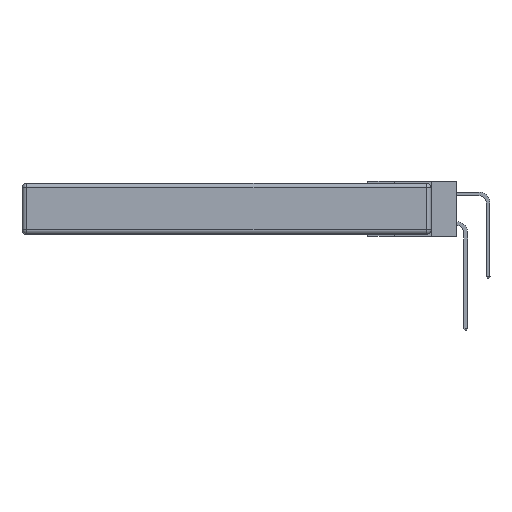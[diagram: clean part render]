
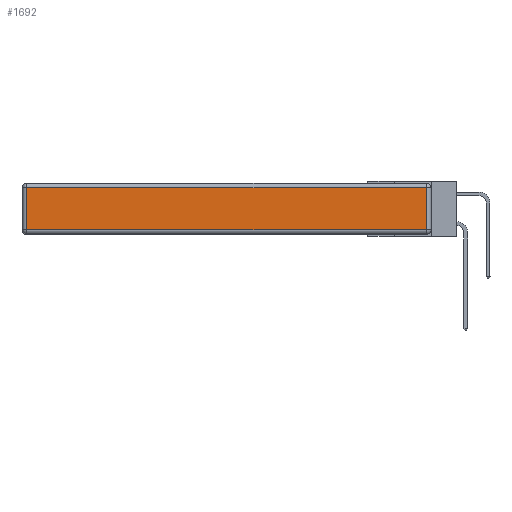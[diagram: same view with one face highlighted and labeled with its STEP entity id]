
A CAD part, left-side view. The second image highlights one B-rep face of the part: STEP entity #1692.
In plain terms, the highlighted planar face has unit normal (-1, 0, 0).
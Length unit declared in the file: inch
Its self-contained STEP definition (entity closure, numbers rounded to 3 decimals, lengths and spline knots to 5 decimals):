
#292 = EDGE_LOOP ( 'NONE', ( #3647, #696, #10602, #1207 ) ) ;
#347 = CARTESIAN_POINT ( 'NONE',  ( 0., 0.03, -0.313 ) ) ;
#696 = ORIENTED_EDGE ( 'NONE', *, *, #6113, .T. ) ;
#996 = PLANE ( 'NONE',  #8773 ) ;
#1207 = ORIENTED_EDGE ( 'NONE', *, *, #12230, .T. ) ;
#1393 = CARTESIAN_POINT ( 'NONE',  ( 0., 0.03, -0.343 ) ) ;
#1673 = DIRECTION ( 'NONE',  ( -1., 0., 0. ) ) ;
#1692 = ADVANCED_FACE ( 'NONE', ( #14883 ), #996, .T. ) ;
#2790 = LINE ( 'NONE', #9106, #5074 ) ;
#3324 = EDGE_CURVE ( 'NONE', #14951, #9114, #3427, .T. ) ;
#3427 = LINE ( 'NONE', #12201, #11537 ) ;
#3623 = VERTEX_POINT ( 'NONE', #14564 ) ;
#3647 = ORIENTED_EDGE ( 'NONE', *, *, #4901, .T. ) ;
#3852 = DIRECTION ( 'NONE',  ( 0., -1., 0. ) ) ;
#4124 = CARTESIAN_POINT ( 'NONE',  ( 0., 0., -0.313 ) ) ;
#4168 = DIRECTION ( 'NONE',  ( 0., 0., 1. ) ) ;
#4195 = CARTESIAN_POINT ( 'NONE',  ( 0., 2.72, -0.03 ) ) ;
#4901 = EDGE_CURVE ( 'NONE', #3623, #14210, #8957, .T. ) ;
#5034 = DIRECTION ( 'NONE',  ( 0., 0., 1. ) ) ;
#5074 = VECTOR ( 'NONE', #14095, 39.37008 ) ;
#5321 = DIRECTION ( 'NONE',  ( 0., 1., 0. ) ) ;
#6113 = EDGE_CURVE ( 'NONE', #14210, #14951, #10579, .T. ) ;
#8773 = AXIS2_PLACEMENT_3D ( 'NONE', #12584, #1673, #4168 ) ;
#8957 = LINE ( 'NONE', #4124, #14773 ) ;
#9106 = CARTESIAN_POINT ( 'NONE',  ( 0., 2.72, -0.343 ) ) ;
#9114 = VERTEX_POINT ( 'NONE', #4195 ) ;
#10579 = LINE ( 'NONE', #1393, #12708 ) ;
#10602 = ORIENTED_EDGE ( 'NONE', *, *, #3324, .T. ) ;
#10802 = CARTESIAN_POINT ( 'NONE',  ( 0., 0.03, -0.03 ) ) ;
#11537 = VECTOR ( 'NONE', #5321, 39.37008 ) ;
#12201 = CARTESIAN_POINT ( 'NONE',  ( 0., 2.75, -0.03 ) ) ;
#12230 = EDGE_CURVE ( 'NONE', #9114, #3623, #2790, .T. ) ;
#12584 = CARTESIAN_POINT ( 'NONE',  ( 0., 0., -0.343 ) ) ;
#12708 = VECTOR ( 'NONE', #5034, 39.37008 ) ;
#14095 = DIRECTION ( 'NONE',  ( 0., 0., -1. ) ) ;
#14210 = VERTEX_POINT ( 'NONE', #347 ) ;
#14564 = CARTESIAN_POINT ( 'NONE',  ( 0., 2.72, -0.313 ) ) ;
#14773 = VECTOR ( 'NONE', #3852, 39.37008 ) ;
#14883 = FACE_OUTER_BOUND ( 'NONE', #292, .T. ) ;
#14951 = VERTEX_POINT ( 'NONE', #10802 ) ;
